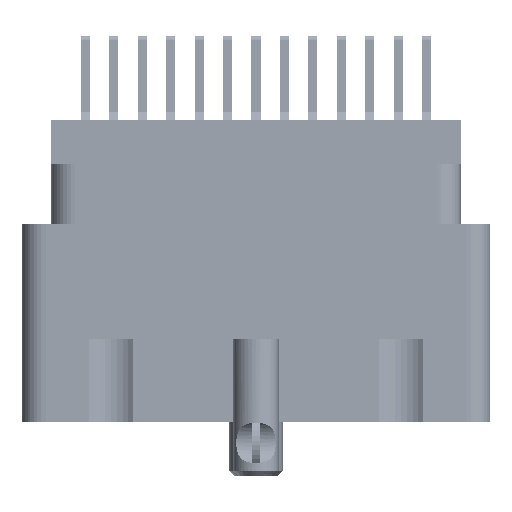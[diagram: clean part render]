
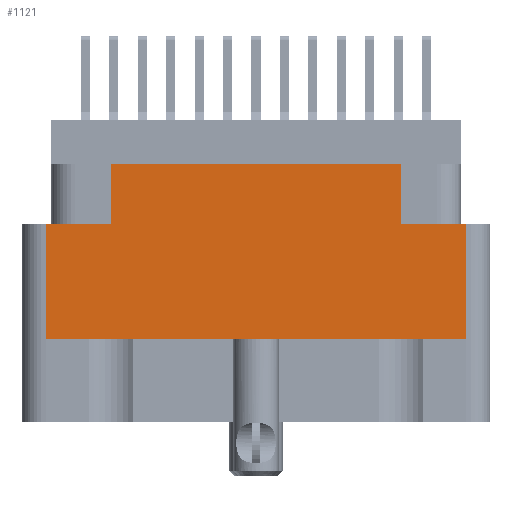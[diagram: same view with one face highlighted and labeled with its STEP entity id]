
A CAD part, left-side view. The second image highlights one B-rep face of the part: STEP entity #1121.
In plain terms, the highlighted planar face has unit normal (-1, 0, 0).
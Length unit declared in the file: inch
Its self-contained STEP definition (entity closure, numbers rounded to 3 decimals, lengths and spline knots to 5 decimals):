
#368 = CARTESIAN_POINT ( 'NONE',  ( -1.359, 0.555, -0.578 ) ) ;
#437 = LINE ( 'NONE', #1663, #56592 ) ;
#445 = ORIENTED_EDGE ( 'NONE', *, *, #55847, .T. ) ;
#1121 = ADVANCED_FACE ( 'NONE', ( #40575 ), #35003, .T. ) ;
#1663 = CARTESIAN_POINT ( 'NONE',  ( -1.359, 0.3825, -0.274 ) ) ;
#1678 = DIRECTION ( 'NONE',  ( 0., -1., 0. ) ) ;
#2279 = VECTOR ( 'NONE', #37259, 39.37008 ) ;
#4888 = EDGE_CURVE ( 'NONE', #6919, #75824, #15487, .T. ) ;
#6636 = AXIS2_PLACEMENT_3D ( 'NONE', #47964, #41628, #28386 ) ;
#6919 = VERTEX_POINT ( 'NONE', #68550 ) ;
#8012 = CARTESIAN_POINT ( 'NONE',  ( -1.359, -0.555, -0.798 ) ) ;
#8066 = LINE ( 'NONE', #69145, #35674 ) ;
#9340 = CARTESIAN_POINT ( 'NONE',  ( -1.359, 0.555, -0.798 ) ) ;
#10582 = CARTESIAN_POINT ( 'NONE',  ( -1.359, -0.3825, -0.274 ) ) ;
#10824 = VERTEX_POINT ( 'NONE', #23200 ) ;
#11373 = EDGE_CURVE ( 'NONE', #28322, #34588, #20403, .T. ) ;
#11528 = VECTOR ( 'NONE', #30074, 39.37008 ) ;
#15487 = LINE ( 'NONE', #10582, #11528 ) ;
#18910 = VECTOR ( 'NONE', #52378, 39.37008 ) ;
#20403 = LINE ( 'NONE', #72219, #49076 ) ;
#22913 = LINE ( 'NONE', #30660, #2279 ) ;
#23200 = CARTESIAN_POINT ( 'NONE',  ( -1.359, -0.555, -0.578 ) ) ;
#24030 = CARTESIAN_POINT ( 'NONE',  ( -1.359, -0.555, -0.274 ) ) ;
#25485 = CARTESIAN_POINT ( 'NONE',  ( -1.359, 0., -0.578 ) ) ;
#26282 = ORIENTED_EDGE ( 'NONE', *, *, #76816, .F. ) ;
#28322 = VERTEX_POINT ( 'NONE', #78545 ) ;
#28386 = DIRECTION ( 'NONE',  ( 0., 0., 1. ) ) ;
#30074 = DIRECTION ( 'NONE',  ( 0., 0., 1. ) ) ;
#30660 = CARTESIAN_POINT ( 'NONE',  ( -1.359, 0.617, -0.117 ) ) ;
#30760 = ORIENTED_EDGE ( 'NONE', *, *, #4888, .T. ) ;
#31699 = LINE ( 'NONE', #8012, #18910 ) ;
#34006 = ORIENTED_EDGE ( 'NONE', *, *, #67905, .F. ) ;
#34588 = VERTEX_POINT ( 'NONE', #66237 ) ;
#34668 = LINE ( 'NONE', #25485, #47518 ) ;
#35003 = PLANE ( 'NONE',  #6636 ) ;
#35674 = VECTOR ( 'NONE', #1678, 39.37008 ) ;
#36880 = EDGE_LOOP ( 'NONE', ( #57119, #69528, #71574, #445, #34006, #30760, #37860, #26282 ) ) ;
#37259 = DIRECTION ( 'NONE',  ( 0., -1., 0. ) ) ;
#37860 = ORIENTED_EDGE ( 'NONE', *, *, #75552, .F. ) ;
#40575 = FACE_OUTER_BOUND ( 'NONE', #36880, .T. ) ;
#41628 = DIRECTION ( 'NONE',  ( -1., 0., 0. ) ) ;
#47518 = VECTOR ( 'NONE', #75686, 39.37008 ) ;
#47964 = CARTESIAN_POINT ( 'NONE',  ( -1.359, -0.617, -0.798 ) ) ;
#49076 = VECTOR ( 'NONE', #60429, 39.37008 ) ;
#52378 = DIRECTION ( 'NONE',  ( 0., 0., 1. ) ) ;
#54395 = VERTEX_POINT ( 'NONE', #65592 ) ;
#55847 = EDGE_CURVE ( 'NONE', #10824, #56724, #31699, .T. ) ;
#56592 = VECTOR ( 'NONE', #58399, 39.37008 ) ;
#56724 = VERTEX_POINT ( 'NONE', #24030 ) ;
#57119 = ORIENTED_EDGE ( 'NONE', *, *, #11373, .F. ) ;
#58399 = DIRECTION ( 'NONE',  ( 0., 0., 1. ) ) ;
#60429 = DIRECTION ( 'NONE',  ( 0., -1., 0. ) ) ;
#65592 = CARTESIAN_POINT ( 'NONE',  ( -1.359, 0.3825, -0.117 ) ) ;
#66083 = DIRECTION ( 'NONE',  ( 0., 0., -1. ) ) ;
#66185 = CARTESIAN_POINT ( 'NONE',  ( -1.359, -0.3825, -0.117 ) ) ;
#66187 = VERTEX_POINT ( 'NONE', #368 ) ;
#66237 = CARTESIAN_POINT ( 'NONE',  ( -1.359, 0.3825, -0.274 ) ) ;
#67905 = EDGE_CURVE ( 'NONE', #6919, #56724, #8066, .T. ) ;
#68550 = CARTESIAN_POINT ( 'NONE',  ( -1.359, -0.3825, -0.274 ) ) ;
#69145 = CARTESIAN_POINT ( 'NONE',  ( -1.359, 0., -0.274 ) ) ;
#69528 = ORIENTED_EDGE ( 'NONE', *, *, #76310, .T. ) ;
#70040 = VECTOR ( 'NONE', #66083, 39.37008 ) ;
#71574 = ORIENTED_EDGE ( 'NONE', *, *, #78369, .T. ) ;
#72219 = CARTESIAN_POINT ( 'NONE',  ( -1.359, 0., -0.274 ) ) ;
#74022 = LINE ( 'NONE', #9340, #70040 ) ;
#75552 = EDGE_CURVE ( 'NONE', #54395, #75824, #22913, .T. ) ;
#75686 = DIRECTION ( 'NONE',  ( 0., -1., 0. ) ) ;
#75824 = VERTEX_POINT ( 'NONE', #66185 ) ;
#76310 = EDGE_CURVE ( 'NONE', #28322, #66187, #74022, .T. ) ;
#76816 = EDGE_CURVE ( 'NONE', #34588, #54395, #437, .T. ) ;
#78369 = EDGE_CURVE ( 'NONE', #66187, #10824, #34668, .T. ) ;
#78545 = CARTESIAN_POINT ( 'NONE',  ( -1.359, 0.555, -0.274 ) ) ;
